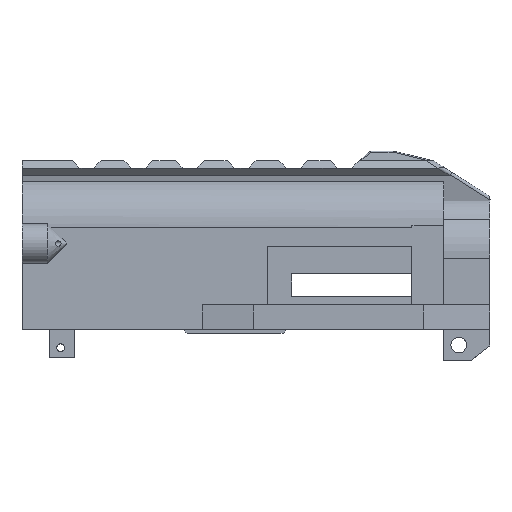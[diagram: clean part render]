
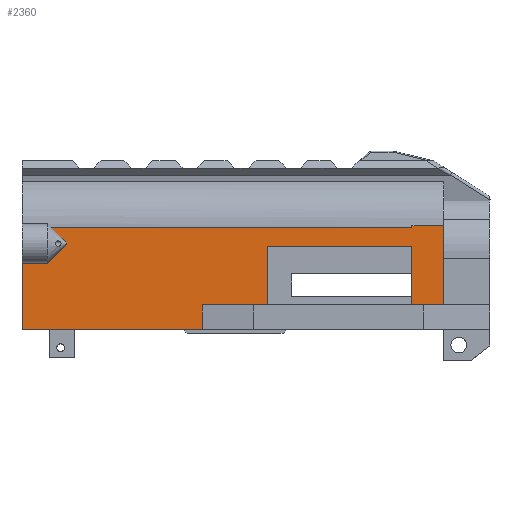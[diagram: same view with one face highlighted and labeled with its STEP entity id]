
A CAD part, top view. The second image highlights one B-rep face of the part: STEP entity #2360.
In plain terms, the highlighted planar face has unit normal (0, 0, 1).
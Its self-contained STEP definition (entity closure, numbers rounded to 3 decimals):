
#139 = VERTEX_POINT ( 'NONE', #6949 ) ;
#268 = EDGE_CURVE ( 'NONE', #4632, #2682, #906, .T. ) ;
#300 = DIRECTION ( 'NONE',  ( -1., 0., 0. ) ) ;
#330 = EDGE_CURVE ( 'NONE', #4414, #9914, #12201, .T. ) ;
#357 = VECTOR ( 'NONE', #13451, 1000. ) ;
#485 = CARTESIAN_POINT ( 'NONE',  ( -19.97, 48.04, 20.1 ) ) ;
#507 = VERTEX_POINT ( 'NONE', #4241 ) ;
#628 = DIRECTION ( 'NONE',  ( 0., 0., 1. ) ) ;
#631 = DIRECTION ( 'NONE',  ( -1., 0., 0. ) ) ;
#675 = EDGE_CURVE ( 'NONE', #5720, #9691, #10841, .T. ) ;
#716 = DIRECTION ( 'NONE',  ( 0., 1., 0. ) ) ;
#813 = CARTESIAN_POINT ( 'NONE',  ( -19.97, 40.076, 20.1 ) ) ;
#906 = LINE ( 'NONE', #485, #4443 ) ;
#986 = DIRECTION ( 'NONE',  ( 1., 0., 0. ) ) ;
#1059 = CARTESIAN_POINT ( 'NONE',  ( -166.91, 48.04, 20.1 ) ) ;
#1073 = EDGE_CURVE ( 'NONE', #9116, #2045, #9990, .T. ) ;
#1079 = ORIENTED_EDGE ( 'NONE', *, *, #10454, .T. ) ;
#1169 = VERTEX_POINT ( 'NONE', #9774 ) ;
#1224 = LINE ( 'NONE', #2760, #357 ) ;
#1269 = CARTESIAN_POINT ( 'NONE',  ( -105.221, 48.04, 20.1 ) ) ;
#1574 = DIRECTION ( 'NONE',  ( 0., -1., 0. ) ) ;
#1596 = LINE ( 'NONE', #1059, #9523 ) ;
#1729 = ORIENTED_EDGE ( 'NONE', *, *, #4819, .F. ) ;
#1736 = CARTESIAN_POINT ( 'NONE',  ( -159.565, 6.49, 20.1 ) ) ;
#1883 = CARTESIAN_POINT ( 'NONE',  ( -19.865, 48.04, 20.1 ) ) ;
#2045 = VERTEX_POINT ( 'NONE', #5712 ) ;
#2184 = DIRECTION ( 'NONE',  ( -0.707, -0.707, 0. ) ) ;
#2222 = CARTESIAN_POINT ( 'NONE',  ( -6.865, 48.66, 20.1 ) ) ;
#2258 = VECTOR ( 'NONE', #11354, 1000. ) ;
#2309 = LINE ( 'NONE', #8701, #2499 ) ;
#2321 = VECTOR ( 'NONE', #5405, 1000. ) ;
#2360 = ADVANCED_FACE ( 'NONE', ( #6890 ), #10378, .T. ) ;
#2499 = VECTOR ( 'NONE', #2184, 1000. ) ;
#2530 = ORIENTED_EDGE ( 'NONE', *, *, #13299, .T. ) ;
#2634 = EDGE_CURVE ( 'NONE', #9691, #1169, #9081, .T. ) ;
#2682 = VERTEX_POINT ( 'NONE', #3262 ) ;
#2758 = VECTOR ( 'NONE', #631, 1000. ) ;
#2760 = CARTESIAN_POINT ( 'NONE',  ( -160.497, 48.04, 20.1 ) ) ;
#2923 = CARTESIAN_POINT ( 'NONE',  ( -105.221, 6.49, 20.1 ) ) ;
#3262 = CARTESIAN_POINT ( 'NONE',  ( -19.97, 16.49, 20.1 ) ) ;
#3478 = CARTESIAN_POINT ( 'NONE',  ( -2.359, 48.66, 20.1 ) ) ;
#3546 = LINE ( 'NONE', #3478, #10280 ) ;
#4000 = VERTEX_POINT ( 'NONE', #2222 ) ;
#4094 = CARTESIAN_POINT ( 'NONE',  ( -6.865, -4.94, 20.1 ) ) ;
#4241 = CARTESIAN_POINT ( 'NONE',  ( -6.865, 16.49, 20.1 ) ) ;
#4410 = ORIENTED_EDGE ( 'NONE', *, *, #268, .T. ) ;
#4414 = VERTEX_POINT ( 'NONE', #4838 ) ;
#4443 = VECTOR ( 'NONE', #1574, 1000. ) ;
#4528 = EDGE_CURVE ( 'NONE', #10440, #4632, #5846, .T. ) ;
#4632 = VERTEX_POINT ( 'NONE', #813 ) ;
#4819 = EDGE_CURVE ( 'NONE', #5720, #6092, #12901, .T. ) ;
#4838 = CARTESIAN_POINT ( 'NONE',  ( -19.865, 48.04, 20.1 ) ) ;
#5039 = CARTESIAN_POINT ( 'NONE',  ( -178.497, 6.49, 20.1 ) ) ;
#5098 = ORIENTED_EDGE ( 'NONE', *, *, #5154, .T. ) ;
#5154 = EDGE_CURVE ( 'NONE', #1169, #10440, #7507, .T. ) ;
#5186 = CARTESIAN_POINT ( 'NONE',  ( -19.865, 33.428, 20.1 ) ) ;
#5283 = ORIENTED_EDGE ( 'NONE', *, *, #2634, .T. ) ;
#5318 = CARTESIAN_POINT ( 'NONE',  ( -19.865, -4.94, 20.1 ) ) ;
#5370 = DIRECTION ( 'NONE',  ( 0., -1., 0. ) ) ;
#5379 = EDGE_CURVE ( 'NONE', #9914, #11900, #1596, .T. ) ;
#5405 = DIRECTION ( 'NONE',  ( 1., 0., 0. ) ) ;
#5712 = CARTESIAN_POINT ( 'NONE',  ( -178.497, 33.428, 20.1 ) ) ;
#5720 = VERTEX_POINT ( 'NONE', #2923 ) ;
#5787 = VECTOR ( 'NONE', #7333, 1000. ) ;
#5805 = EDGE_CURVE ( 'NONE', #2045, #6092, #10870, .T. ) ;
#5846 = LINE ( 'NONE', #11415, #11217 ) ;
#6092 = VERTEX_POINT ( 'NONE', #5039 ) ;
#6199 = ORIENTED_EDGE ( 'NONE', *, *, #9055, .T. ) ;
#6890 = FACE_OUTER_BOUND ( 'NONE', #8266, .T. ) ;
#6949 = CARTESIAN_POINT ( 'NONE',  ( -19.865, 48.66, 20.1 ) ) ;
#6980 = EDGE_CURVE ( 'NONE', #507, #4000, #7816, .T. ) ;
#7120 = VECTOR ( 'NONE', #5370, 1000. ) ;
#7194 = ORIENTED_EDGE ( 'NONE', *, *, #330, .T. ) ;
#7210 = DIRECTION ( 'NONE',  ( 0., -1., 0. ) ) ;
#7333 = DIRECTION ( 'NONE',  ( -1., 0., 0. ) ) ;
#7469 = DIRECTION ( 'NONE',  ( 0., 1., 0. ) ) ;
#7507 = LINE ( 'NONE', #10421, #11382 ) ;
#7760 = CARTESIAN_POINT ( 'NONE',  ( -160.497, 41.228, 20.1 ) ) ;
#7816 = LINE ( 'NONE', #4094, #11536 ) ;
#8190 = VERTEX_POINT ( 'NONE', #7760 ) ;
#8266 = EDGE_LOOP ( 'NONE', ( #5283, #5098, #9464, #4410, #9110, #9515, #8491, #1079, #7194, #13830, #6199, #2530, #10036, #10477, #1729, #10772 ) ) ;
#8331 = VECTOR ( 'NONE', #7210, 1000. ) ;
#8491 = ORIENTED_EDGE ( 'NONE', *, *, #12237, .T. ) ;
#8701 = CARTESIAN_POINT ( 'NONE',  ( -160.497, 41.228, 20.1 ) ) ;
#9055 = EDGE_CURVE ( 'NONE', #11900, #8190, #1224, .T. ) ;
#9081 = LINE ( 'NONE', #10887, #2321 ) ;
#9110 = ORIENTED_EDGE ( 'NONE', *, *, #12025, .T. ) ;
#9116 = VERTEX_POINT ( 'NONE', #10290 ) ;
#9311 = LINE ( 'NONE', #5318, #7120 ) ;
#9328 = VECTOR ( 'NONE', #9843, 1000. ) ;
#9464 = ORIENTED_EDGE ( 'NONE', *, *, #4528, .T. ) ;
#9515 = ORIENTED_EDGE ( 'NONE', *, *, #6980, .T. ) ;
#9523 = VECTOR ( 'NONE', #13968, 1000. ) ;
#9624 = AXIS2_PLACEMENT_3D ( 'NONE', #1883, #628, #13666 ) ;
#9691 = VERTEX_POINT ( 'NONE', #11532 ) ;
#9747 = CARTESIAN_POINT ( 'NONE',  ( -166.91, 48.04, 20.1 ) ) ;
#9774 = CARTESIAN_POINT ( 'NONE',  ( -78.815, 16.49, 20.1 ) ) ;
#9843 = DIRECTION ( 'NONE',  ( 0., 1., 0. ) ) ;
#9914 = VERTEX_POINT ( 'NONE', #9747 ) ;
#9990 = LINE ( 'NONE', #5186, #5787 ) ;
#10036 = ORIENTED_EDGE ( 'NONE', *, *, #1073, .T. ) ;
#10280 = VECTOR ( 'NONE', #300, 1000. ) ;
#10290 = CARTESIAN_POINT ( 'NONE',  ( -168.297, 33.428, 20.1 ) ) ;
#10378 = PLANE ( 'NONE',  #9624 ) ;
#10421 = CARTESIAN_POINT ( 'NONE',  ( -78.815, 48.04, 20.1 ) ) ;
#10440 = VERTEX_POINT ( 'NONE', #11793 ) ;
#10454 = EDGE_CURVE ( 'NONE', #139, #4414, #9311, .T. ) ;
#10477 = ORIENTED_EDGE ( 'NONE', *, *, #5805, .T. ) ;
#10772 = ORIENTED_EDGE ( 'NONE', *, *, #675, .T. ) ;
#10841 = LINE ( 'NONE', #1269, #9328 ) ;
#10870 = LINE ( 'NONE', #12534, #8331 ) ;
#10887 = CARTESIAN_POINT ( 'NONE',  ( -19.865, 16.49, 20.1 ) ) ;
#11217 = VECTOR ( 'NONE', #12357, 1000. ) ;
#11354 = DIRECTION ( 'NONE',  ( -1., 0., 0. ) ) ;
#11382 = VECTOR ( 'NONE', #716, 1000. ) ;
#11415 = CARTESIAN_POINT ( 'NONE',  ( -19.865, 40.076, 20.1 ) ) ;
#11532 = CARTESIAN_POINT ( 'NONE',  ( -105.221, 16.49, 20.1 ) ) ;
#11536 = VECTOR ( 'NONE', #7469, 1000. ) ;
#11723 = CARTESIAN_POINT ( 'NONE',  ( -160.497, 41.628, 20.1 ) ) ;
#11793 = CARTESIAN_POINT ( 'NONE',  ( -78.815, 40.076, 20.1 ) ) ;
#11900 = VERTEX_POINT ( 'NONE', #11723 ) ;
#12025 = EDGE_CURVE ( 'NONE', #2682, #507, #13315, .T. ) ;
#12201 = LINE ( 'NONE', #12499, #2758 ) ;
#12237 = EDGE_CURVE ( 'NONE', #4000, #139, #3546, .T. ) ;
#12357 = DIRECTION ( 'NONE',  ( 1., 0., 0. ) ) ;
#12499 = CARTESIAN_POINT ( 'NONE',  ( -19.865, 48.04, 20.1 ) ) ;
#12534 = CARTESIAN_POINT ( 'NONE',  ( -178.497, 48.04, 20.1 ) ) ;
#12901 = LINE ( 'NONE', #1736, #2258 ) ;
#12947 = CARTESIAN_POINT ( 'NONE',  ( -19.865, 16.49, 20.1 ) ) ;
#13299 = EDGE_CURVE ( 'NONE', #8190, #9116, #2309, .T. ) ;
#13315 = LINE ( 'NONE', #12947, #13647 ) ;
#13451 = DIRECTION ( 'NONE',  ( 0., -1., 0. ) ) ;
#13647 = VECTOR ( 'NONE', #986, 1000. ) ;
#13666 = DIRECTION ( 'NONE',  ( 1., 0., 0. ) ) ;
#13830 = ORIENTED_EDGE ( 'NONE', *, *, #5379, .T. ) ;
#13968 = DIRECTION ( 'NONE',  ( 0.707, -0.707, 0. ) ) ;
